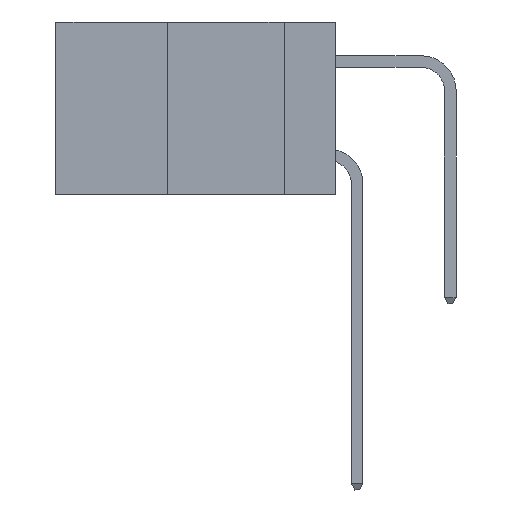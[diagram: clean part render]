
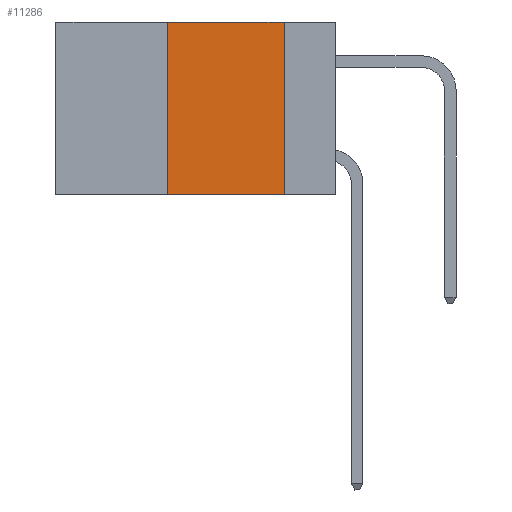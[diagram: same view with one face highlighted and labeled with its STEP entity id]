
A CAD part, left-side view. The second image highlights one B-rep face of the part: STEP entity #11286.
In plain terms, the highlighted planar face has unit normal (-1, 0, 0).
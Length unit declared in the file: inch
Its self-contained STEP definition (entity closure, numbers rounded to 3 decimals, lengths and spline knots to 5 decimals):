
#1824 = CARTESIAN_POINT ( 'NONE',  ( 0., 0.11, 0. ) ) ;
#2165 = VECTOR ( 'NONE', #18548, 39.37008 ) ;
#3297 = CARTESIAN_POINT ( 'NONE',  ( 0., 0.6, -0.37 ) ) ;
#3845 = EDGE_CURVE ( 'NONE', #22182, #23510, #29333, .T. ) ;
#4631 = VECTOR ( 'NONE', #24542, 39.37008 ) ;
#4852 = EDGE_CURVE ( 'NONE', #27258, #23510, #28009, .T. ) ;
#4934 = VECTOR ( 'NONE', #8114, 39.37008 ) ;
#7486 = DIRECTION ( 'NONE',  ( 0., 0., -1. ) ) ;
#7697 = CARTESIAN_POINT ( 'NONE',  ( 0., 0.36, 0. ) ) ;
#8114 = DIRECTION ( 'NONE',  ( 0., -1., 0. ) ) ;
#9260 = EDGE_CURVE ( 'NONE', #12609, #27258, #10486, .T. ) ;
#10308 = LINE ( 'NONE', #19754, #4631 ) ;
#10486 = LINE ( 'NONE', #24732, #21051 ) ;
#10653 = DIRECTION ( 'NONE',  ( 0., -1., 0. ) ) ;
#10866 = EDGE_LOOP ( 'NONE', ( #12042, #19263, #25475, #14552 ) ) ;
#11246 = AXIS2_PLACEMENT_3D ( 'NONE', #25757, #25611, #7486 ) ;
#11286 = ADVANCED_FACE ( 'NONE', ( #14164 ), #28260, .F. ) ;
#12042 = ORIENTED_EDGE ( 'NONE', *, *, #4852, .F. ) ;
#12609 = VERTEX_POINT ( 'NONE', #7697 ) ;
#14164 = FACE_OUTER_BOUND ( 'NONE', #10866, .T. ) ;
#14552 = ORIENTED_EDGE ( 'NONE', *, *, #3845, .T. ) ;
#18548 = DIRECTION ( 'NONE',  ( 0., 0., -1. ) ) ;
#19263 = ORIENTED_EDGE ( 'NONE', *, *, #9260, .F. ) ;
#19754 = CARTESIAN_POINT ( 'NONE',  ( 0., 0.36, 0. ) ) ;
#20351 = EDGE_CURVE ( 'NONE', #22182, #12609, #10308, .T. ) ;
#21051 = VECTOR ( 'NONE', #10653, 39.37008 ) ;
#22182 = VERTEX_POINT ( 'NONE', #25131 ) ;
#23201 = CARTESIAN_POINT ( 'NONE',  ( 0., 0.11, 0. ) ) ;
#23510 = VERTEX_POINT ( 'NONE', #27342 ) ;
#24542 = DIRECTION ( 'NONE',  ( 0., 0., 1. ) ) ;
#24732 = CARTESIAN_POINT ( 'NONE',  ( 0., 0.6, 0. ) ) ;
#25131 = CARTESIAN_POINT ( 'NONE',  ( 0., 0.36, -0.37 ) ) ;
#25475 = ORIENTED_EDGE ( 'NONE', *, *, #20351, .F. ) ;
#25611 = DIRECTION ( 'NONE',  ( 1., 0., 0. ) ) ;
#25757 = CARTESIAN_POINT ( 'NONE',  ( 0., 0.6, 0. ) ) ;
#27258 = VERTEX_POINT ( 'NONE', #1824 ) ;
#27342 = CARTESIAN_POINT ( 'NONE',  ( 0., 0.11, -0.37 ) ) ;
#28009 = LINE ( 'NONE', #23201, #2165 ) ;
#28260 = PLANE ( 'NONE',  #11246 ) ;
#29333 = LINE ( 'NONE', #3297, #4934 ) ;
